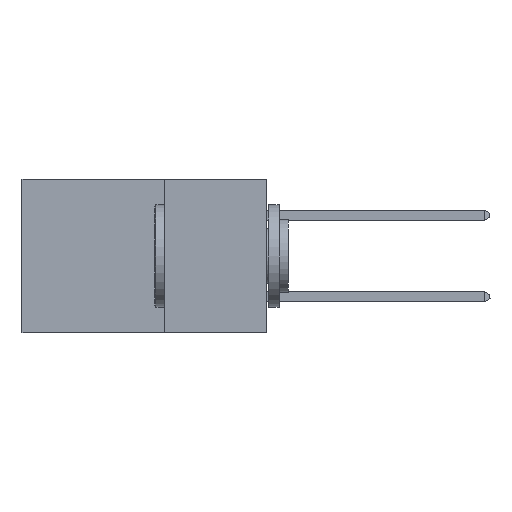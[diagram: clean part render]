
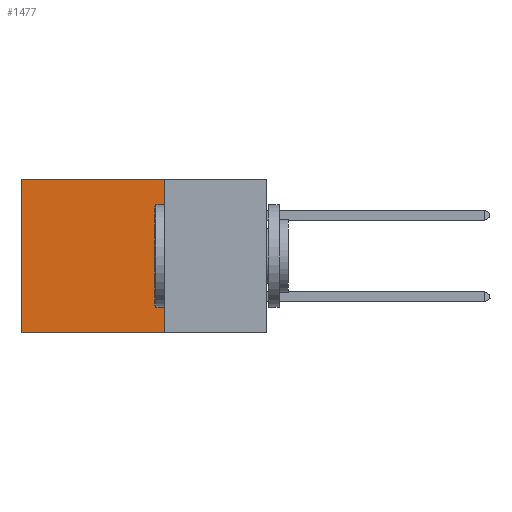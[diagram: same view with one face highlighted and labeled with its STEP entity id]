
A CAD part, left-side view. The second image highlights one B-rep face of the part: STEP entity #1477.
In plain terms, the highlighted planar face has unit normal (-1, 0, 0).
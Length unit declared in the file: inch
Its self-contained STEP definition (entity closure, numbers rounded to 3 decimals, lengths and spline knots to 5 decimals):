
#33 = EDGE_LOOP ( 'NONE', ( #1459, #11958, #14704, #10250 ) ) ;
#207 = CARTESIAN_POINT ( 'NONE',  ( 0.2875, 0.6, 0. ) ) ;
#725 = LINE ( 'NONE', #1161, #13764 ) ;
#1161 = CARTESIAN_POINT ( 'NONE',  ( 0.2875, 0.25, -0.375 ) ) ;
#1205 = DIRECTION ( 'NONE',  ( 0., 1., 0. ) ) ;
#1459 = ORIENTED_EDGE ( 'NONE', *, *, #5445, .T. ) ;
#1477 = ADVANCED_FACE ( 'NONE', ( #2812 ), #5531, .F. ) ;
#1588 = DIRECTION ( 'NONE',  ( 0., 0., -1. ) ) ;
#1607 = CARTESIAN_POINT ( 'NONE',  ( 0.2875, 0.25, 0. ) ) ;
#2004 = CARTESIAN_POINT ( 'NONE',  ( 0.2875, 0.25, 0. ) ) ;
#2812 = FACE_OUTER_BOUND ( 'NONE', #33, .T. ) ;
#2836 = EDGE_CURVE ( 'NONE', #9639, #3000, #3958, .T. ) ;
#3000 = VERTEX_POINT ( 'NONE', #5632 ) ;
#3958 = LINE ( 'NONE', #4133, #4375 ) ;
#4127 = DIRECTION ( 'NONE',  ( 1., 0., 0. ) ) ;
#4133 = CARTESIAN_POINT ( 'NONE',  ( 0.2875, 0.25, -0.375 ) ) ;
#4375 = VECTOR ( 'NONE', #1588, 39.37008 ) ;
#4413 = VECTOR ( 'NONE', #14517, 39.37008 ) ;
#5297 = VERTEX_POINT ( 'NONE', #207 ) ;
#5356 = DIRECTION ( 'NONE',  ( 0., 0., -1. ) ) ;
#5445 = EDGE_CURVE ( 'NONE', #5297, #8190, #5692, .T. ) ;
#5531 = PLANE ( 'NONE',  #8976 ) ;
#5632 = CARTESIAN_POINT ( 'NONE',  ( 0.2875, 0.25, -0.375 ) ) ;
#5692 = LINE ( 'NONE', #14968, #11961 ) ;
#7532 = EDGE_CURVE ( 'NONE', #3000, #8190, #725, .T. ) ;
#7893 = CARTESIAN_POINT ( 'NONE',  ( 0.2875, 0.25, -0.375 ) ) ;
#8190 = VERTEX_POINT ( 'NONE', #8934 ) ;
#8595 = DIRECTION ( 'NONE',  ( 0., 0., -1. ) ) ;
#8934 = CARTESIAN_POINT ( 'NONE',  ( 0.2875, 0.6, -0.375 ) ) ;
#8976 = AXIS2_PLACEMENT_3D ( 'NONE', #7893, #4127, #5356 ) ;
#9639 = VERTEX_POINT ( 'NONE', #1607 ) ;
#9726 = EDGE_CURVE ( 'NONE', #9639, #5297, #15282, .T. ) ;
#10250 = ORIENTED_EDGE ( 'NONE', *, *, #9726, .T. ) ;
#11958 = ORIENTED_EDGE ( 'NONE', *, *, #7532, .F. ) ;
#11961 = VECTOR ( 'NONE', #8595, 39.37008 ) ;
#13764 = VECTOR ( 'NONE', #1205, 39.37008 ) ;
#14517 = DIRECTION ( 'NONE',  ( 0., 1., 0. ) ) ;
#14704 = ORIENTED_EDGE ( 'NONE', *, *, #2836, .F. ) ;
#14968 = CARTESIAN_POINT ( 'NONE',  ( 0.2875, 0.6, -0.375 ) ) ;
#15282 = LINE ( 'NONE', #2004, #4413 ) ;
